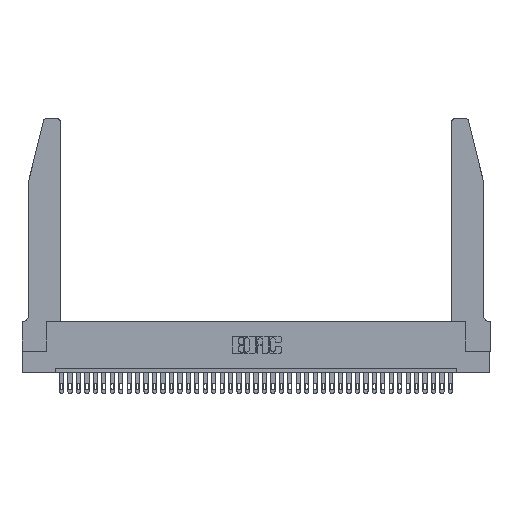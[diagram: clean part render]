
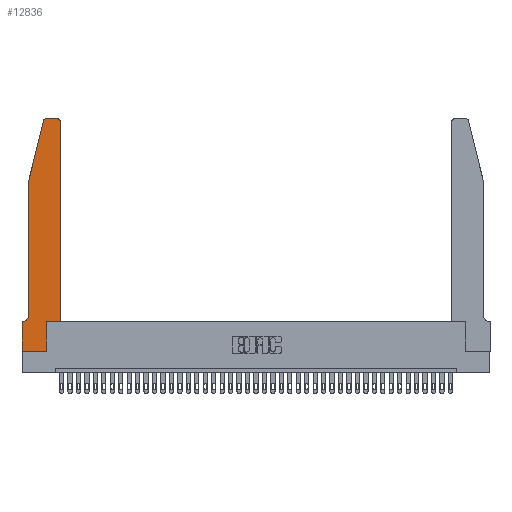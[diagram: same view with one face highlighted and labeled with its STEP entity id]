
A CAD part, top view. The second image highlights one B-rep face of the part: STEP entity #12836.
In plain terms, the highlighted planar face has unit normal (0, 0, 1).
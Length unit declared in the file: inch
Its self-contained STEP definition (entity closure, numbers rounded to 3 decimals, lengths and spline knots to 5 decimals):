
#17 = VERTEX_POINT ( 'NONE', #18788 ) ;
#60 = CARTESIAN_POINT ( 'NONE',  ( 0.2605, 2.75, 0.37 ) ) ;
#218 = CARTESIAN_POINT ( 'NONE',  ( 0.2865, 0., 0.37 ) ) ;
#771 = VECTOR ( 'NONE', #32152, 39.37008 ) ;
#863 = EDGE_CURVE ( 'NONE', #29011, #36873, #22348, .T. ) ;
#1115 = ORIENTED_EDGE ( 'NONE', *, *, #2274, .T. ) ;
#2274 = EDGE_CURVE ( 'NONE', #21147, #35667, #35543, .T. ) ;
#2449 = CARTESIAN_POINT ( 'NONE',  ( 0.0755, 2., 0.37 ) ) ;
#3105 = DIRECTION ( 'NONE',  ( -1., 0., 0. ) ) ;
#3982 = VECTOR ( 'NONE', #11723, 39.37008 ) ;
#5171 = LINE ( 'NONE', #34180, #38481 ) ;
#5587 = ORIENTED_EDGE ( 'NONE', *, *, #29587, .T. ) ;
#5673 = LINE ( 'NONE', #21740, #10407 ) ;
#5965 = CARTESIAN_POINT ( 'NONE',  ( 0.4505, 0.35, 0.37 ) ) ;
#6025 = DIRECTION ( 'NONE',  ( 1., 0., 0. ) ) ;
#6763 = CARTESIAN_POINT ( 'NONE',  ( 0.0755, 0.42, 0.37 ) ) ;
#7395 = CARTESIAN_POINT ( 'NONE',  ( 0., 0.35, 0.37 ) ) ;
#7912 = DIRECTION ( 'NONE',  ( -1., 0., 0. ) ) ;
#8548 = CARTESIAN_POINT ( 'NONE',  ( 0.25487, 2.72718, 0.37 ) ) ;
#8669 = ORIENTED_EDGE ( 'NONE', *, *, #23738, .T. ) ;
#8694 = DIRECTION ( 'NONE',  ( 1., 0., 0. ) ) ;
#8953 = ORIENTED_EDGE ( 'NONE', *, *, #27420, .T. ) ;
#9748 = EDGE_CURVE ( 'NONE', #17, #19808, #29111, .T. ) ;
#9818 = ORIENTED_EDGE ( 'NONE', *, *, #9748, .T. ) ;
#10407 = VECTOR ( 'NONE', #24523, 39.37008 ) ;
#10499 = VECTOR ( 'NONE', #29161, 39.37008 ) ;
#10883 = CARTESIAN_POINT ( 'NONE',  ( 0., 0., 0.37 ) ) ;
#11723 = DIRECTION ( 'NONE',  ( 0., 1., 0. ) ) ;
#12226 = EDGE_CURVE ( 'NONE', #19808, #38574, #5171, .T. ) ;
#12363 = VERTEX_POINT ( 'NONE', #6763 ) ;
#12542 = EDGE_CURVE ( 'NONE', #12363, #37292, #28934, .T. ) ;
#12580 = LINE ( 'NONE', #20838, #20723 ) ;
#12836 = ADVANCED_FACE ( 'NONE', ( #35567 ), #17361, .T. ) ;
#13531 = AXIS2_PLACEMENT_3D ( 'NONE', #33047, #30743, #6025 ) ;
#14322 = ORIENTED_EDGE ( 'NONE', *, *, #20048, .T. ) ;
#14433 = EDGE_LOOP ( 'NONE', ( #5587, #9818, #14912, #8669, #27790, #8953, #1115, #17372, #26615, #25067, #14322, #38770 ) ) ;
#14912 = ORIENTED_EDGE ( 'NONE', *, *, #12226, .T. ) ;
#15583 = EDGE_CURVE ( 'NONE', #35667, #36909, #29564, .T. ) ;
#16324 = DIRECTION ( 'NONE',  ( 1., 0., 0. ) ) ;
#17360 = VECTOR ( 'NONE', #26739, 39.37008 ) ;
#17361 = PLANE ( 'NONE',  #13531 ) ;
#17372 = ORIENTED_EDGE ( 'NONE', *, *, #15583, .T. ) ;
#17578 = CARTESIAN_POINT ( 'NONE',  ( 0.2865, 0.35, 0.37 ) ) ;
#17734 = AXIS2_PLACEMENT_3D ( 'NONE', #34692, #37889, #16324 ) ;
#17822 = LINE ( 'NONE', #5965, #17360 ) ;
#18285 = CARTESIAN_POINT ( 'NONE',  ( 0.4205, 2.75, 0.37 ) ) ;
#18788 = CARTESIAN_POINT ( 'NONE',  ( 0.284, 2.75, 0.37 ) ) ;
#18907 = VECTOR ( 'NONE', #7912, 39.37008 ) ;
#19003 = DIRECTION ( 'NONE',  ( -0.239, -0.971, 0. ) ) ;
#19712 = VECTOR ( 'NONE', #3105, 39.37008 ) ;
#19808 = VERTEX_POINT ( 'NONE', #8548 ) ;
#20048 = EDGE_CURVE ( 'NONE', #24189, #29011, #17822, .T. ) ;
#20273 = EDGE_CURVE ( 'NONE', #36909, #29026, #30612, .T. ) ;
#20458 = DIRECTION ( 'NONE',  ( 1., 0., 0. ) ) ;
#20723 = VECTOR ( 'NONE', #8694, 39.37008 ) ;
#20727 = DIRECTION ( 'NONE',  ( 0., 0., 1. ) ) ;
#20838 = CARTESIAN_POINT ( 'NONE',  ( 0.4505, 0.35, 0.37 ) ) ;
#21147 = VERTEX_POINT ( 'NONE', #7395 ) ;
#21740 = CARTESIAN_POINT ( 'NONE',  ( 0.0755, 2., 0.37 ) ) ;
#21845 = AXIS2_PLACEMENT_3D ( 'NONE', #32691, #20727, #20458 ) ;
#22139 = CARTESIAN_POINT ( 'NONE',  ( 0.4505, 0.35, 0.37 ) ) ;
#22192 = AXIS2_PLACEMENT_3D ( 'NONE', #24320, #27409, #33157 ) ;
#22348 = CIRCLE ( 'NONE', #21845, 0.03 ) ;
#23738 = EDGE_CURVE ( 'NONE', #38574, #12363, #5673, .T. ) ;
#24153 = LINE ( 'NONE', #29330, #18907 ) ;
#24189 = VERTEX_POINT ( 'NONE', #22139 ) ;
#24320 = CARTESIAN_POINT ( 'NONE',  ( 0.0055, 0.42, 0.37 ) ) ;
#24523 = DIRECTION ( 'NONE',  ( 0., -1., 0. ) ) ;
#24899 = CARTESIAN_POINT ( 'NONE',  ( 0.2865, 0.35, 0.37 ) ) ;
#25067 = ORIENTED_EDGE ( 'NONE', *, *, #26071, .T. ) ;
#26071 = EDGE_CURVE ( 'NONE', #29026, #24189, #12580, .T. ) ;
#26615 = ORIENTED_EDGE ( 'NONE', *, *, #20273, .T. ) ;
#26739 = DIRECTION ( 'NONE',  ( 0., 1., 0. ) ) ;
#27409 = DIRECTION ( 'NONE',  ( 0., 0., -1. ) ) ;
#27420 = EDGE_CURVE ( 'NONE', #37292, #21147, #24153, .T. ) ;
#27790 = ORIENTED_EDGE ( 'NONE', *, *, #12542, .T. ) ;
#28934 = CIRCLE ( 'NONE', #22192, 0.07 ) ;
#29011 = VERTEX_POINT ( 'NONE', #36258 ) ;
#29026 = VERTEX_POINT ( 'NONE', #24899 ) ;
#29111 = CIRCLE ( 'NONE', #17734, 0.03 ) ;
#29161 = DIRECTION ( 'NONE',  ( 1., 0., 0. ) ) ;
#29266 = CARTESIAN_POINT ( 'NONE',  ( 0.0055, 0.35, 0.37 ) ) ;
#29330 = CARTESIAN_POINT ( 'NONE',  ( 0.0755, 0.35, 0.37 ) ) ;
#29557 = CARTESIAN_POINT ( 'NONE',  ( 0., 0., 0.37 ) ) ;
#29564 = LINE ( 'NONE', #29557, #10499 ) ;
#29587 = EDGE_CURVE ( 'NONE', #36873, #17, #36824, .T. ) ;
#30612 = LINE ( 'NONE', #17578, #3982 ) ;
#30743 = DIRECTION ( 'NONE',  ( 0., 0., 1. ) ) ;
#32152 = DIRECTION ( 'NONE',  ( 0., -1., 0. ) ) ;
#32691 = CARTESIAN_POINT ( 'NONE',  ( 0.4205, 2.72, 0.37 ) ) ;
#33047 = CARTESIAN_POINT ( 'NONE',  ( 0., 0.35, 0.37 ) ) ;
#33157 = DIRECTION ( 'NONE',  ( -1., 0., 0. ) ) ;
#34180 = CARTESIAN_POINT ( 'NONE',  ( 0.0755, 2., 0.37 ) ) ;
#34692 = CARTESIAN_POINT ( 'NONE',  ( 0.284, 2.72, 0.37 ) ) ;
#35543 = LINE ( 'NONE', #10883, #771 ) ;
#35567 = FACE_OUTER_BOUND ( 'NONE', #14433, .T. ) ;
#35667 = VERTEX_POINT ( 'NONE', #36806 ) ;
#36258 = CARTESIAN_POINT ( 'NONE',  ( 0.4505, 2.72, 0.37 ) ) ;
#36806 = CARTESIAN_POINT ( 'NONE',  ( 0., 0., 0.37 ) ) ;
#36824 = LINE ( 'NONE', #60, #19712 ) ;
#36873 = VERTEX_POINT ( 'NONE', #18285 ) ;
#36909 = VERTEX_POINT ( 'NONE', #218 ) ;
#37292 = VERTEX_POINT ( 'NONE', #29266 ) ;
#37889 = DIRECTION ( 'NONE',  ( 0., 0., 1. ) ) ;
#38481 = VECTOR ( 'NONE', #19003, 39.37008 ) ;
#38574 = VERTEX_POINT ( 'NONE', #2449 ) ;
#38770 = ORIENTED_EDGE ( 'NONE', *, *, #863, .T. ) ;
